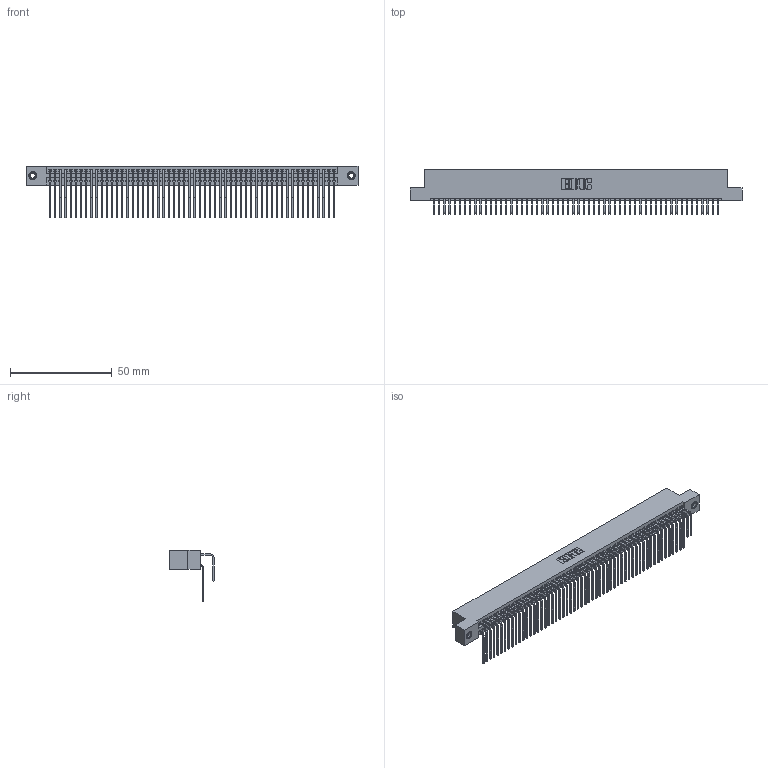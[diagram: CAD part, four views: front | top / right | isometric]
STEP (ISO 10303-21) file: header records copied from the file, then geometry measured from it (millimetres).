
FILE_DESCRIPTION (( 'STEP AP203' ), '1' );
FILE_NAME ('395-112-558-207.STEP', '2018-12-01T11:59:41', ( '' ), ( '' ), 'SwSTEP 2.0', 'SolidWorks 2016', '' );
FILE_SCHEMA (( 'CONFIG_CONTROL_DESIGN' ));
Length unit declared in the file: inch
Products named in the file (5): 345-250-001_345-250-005-103; 345-292-001_558 Tail - 2; 345-292-001_558 559 Tail - 1; 395-112-558-207; 345 Part_Flush Mounting Lugs - 0.156 Dia-TI
Assembly tree (115 placements, depth 2):
  395-112-558-207
    345 Part_Flush Mounting Lugs - 0.156 Dia-TI
    345-292-001_558 559 Tail - 1  x56
    345-292-001_558 Tail - 2  x56
    345-250-001_345-250-005-103  x2
Bounding box: 163.45 x 21.83 x 25.53 mm (x, y, z)
Volume: 16640.1 mm3; surface area: 27934.1 mm2
Topology: 115 solids, 115 shells, 6010 faces, 17837 edges, 11734 vertices
Faces by surface type: plane 4032, cylinder 1962, cone 12, torus 4
Entity records: 44892 total; most frequent: CARTESIAN_POINT 7538, ORIENTED_EDGE 7414, DIRECTION 6629, EDGE_CURVE 3707, LINE 3291, VECTOR 3291, VERTEX_POINT 2464, AXIS2_PLACEMENT_3D 1669
